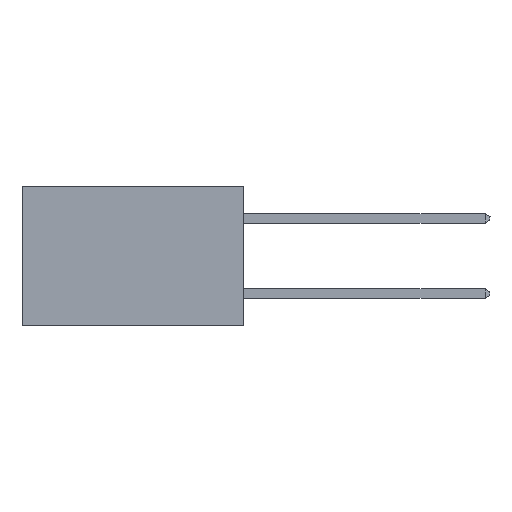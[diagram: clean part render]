
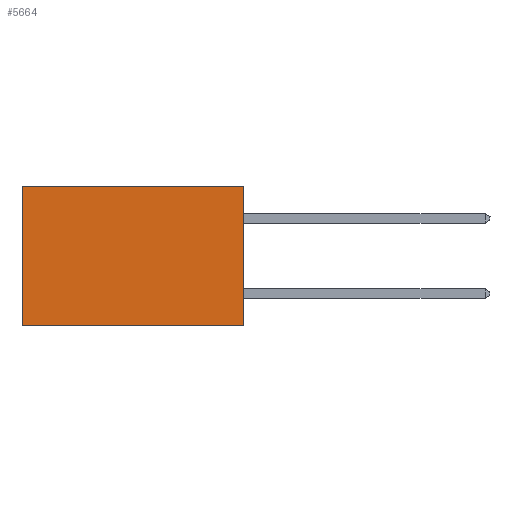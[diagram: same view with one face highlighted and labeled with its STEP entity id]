
A CAD part, left-side view. The second image highlights one B-rep face of the part: STEP entity #5664.
In plain terms, the highlighted planar face has unit normal (-1, 0, 0).
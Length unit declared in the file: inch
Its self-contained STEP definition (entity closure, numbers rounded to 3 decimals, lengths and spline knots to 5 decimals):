
#2403 = DIRECTION ( 'NONE',  ( 0., 0., -1. ) ) ;
#3156 = ORIENTED_EDGE ( 'NONE', *, *, #4374, .F. ) ;
#3674 = DIRECTION ( 'NONE',  ( 0., 0., -1. ) ) ;
#3703 = DIRECTION ( 'NONE',  ( 1., 0., 0. ) ) ;
#3738 = PLANE ( 'NONE',  #9442 ) ;
#3856 = LINE ( 'NONE', #19989, #17096 ) ;
#3900 = EDGE_LOOP ( 'NONE', ( #17057, #3156, #21816, #6481 ) ) ;
#4192 = VERTEX_POINT ( 'NONE', #14874 ) ;
#4220 = CARTESIAN_POINT ( 'NONE',  ( 0.277, 0., -0.37 ) ) ;
#4374 = EDGE_CURVE ( 'NONE', #10884, #13451, #4929, .T. ) ;
#4837 = EDGE_CURVE ( 'NONE', #24887, #4192, #20628, .T. ) ;
#4929 = LINE ( 'NONE', #12263, #15275 ) ;
#5664 = ADVANCED_FACE ( 'NONE', ( #12331 ), #3738, .F. ) ;
#6481 = ORIENTED_EDGE ( 'NONE', *, *, #4837, .T. ) ;
#6520 = DIRECTION ( 'NONE',  ( 0., 1., 0. ) ) ;
#6701 = CARTESIAN_POINT ( 'NONE',  ( 0.277, 0., 0. ) ) ;
#7047 = CARTESIAN_POINT ( 'NONE',  ( 0.277, 0., 0. ) ) ;
#9116 = CARTESIAN_POINT ( 'NONE',  ( 0.277, 0., -0.37 ) ) ;
#9442 = AXIS2_PLACEMENT_3D ( 'NONE', #4220, #3703, #3674 ) ;
#10814 = LINE ( 'NONE', #18863, #25779 ) ;
#10884 = VERTEX_POINT ( 'NONE', #9116 ) ;
#11320 = CARTESIAN_POINT ( 'NONE',  ( 0.277, 0.59, -0.37 ) ) ;
#12194 = DIRECTION ( 'NONE',  ( 0., 1., 0. ) ) ;
#12263 = CARTESIAN_POINT ( 'NONE',  ( 0.277, 0., -0.37 ) ) ;
#12331 = FACE_OUTER_BOUND ( 'NONE', #3900, .T. ) ;
#13451 = VERTEX_POINT ( 'NONE', #11320 ) ;
#14874 = CARTESIAN_POINT ( 'NONE',  ( 0.277, 0.59, 0. ) ) ;
#15251 = VECTOR ( 'NONE', #6520, 39.37008 ) ;
#15275 = VECTOR ( 'NONE', #12194, 39.37008 ) ;
#17057 = ORIENTED_EDGE ( 'NONE', *, *, #17772, .T. ) ;
#17096 = VECTOR ( 'NONE', #22131, 39.37008 ) ;
#17772 = EDGE_CURVE ( 'NONE', #4192, #13451, #3856, .T. ) ;
#18863 = CARTESIAN_POINT ( 'NONE',  ( 0.277, 0., -0.37 ) ) ;
#19989 = CARTESIAN_POINT ( 'NONE',  ( 0.277, 0.59, -0.37 ) ) ;
#20628 = LINE ( 'NONE', #6701, #15251 ) ;
#21816 = ORIENTED_EDGE ( 'NONE', *, *, #25474, .F. ) ;
#22131 = DIRECTION ( 'NONE',  ( 0., 0., -1. ) ) ;
#24887 = VERTEX_POINT ( 'NONE', #7047 ) ;
#25474 = EDGE_CURVE ( 'NONE', #24887, #10884, #10814, .T. ) ;
#25779 = VECTOR ( 'NONE', #2403, 39.37008 ) ;
